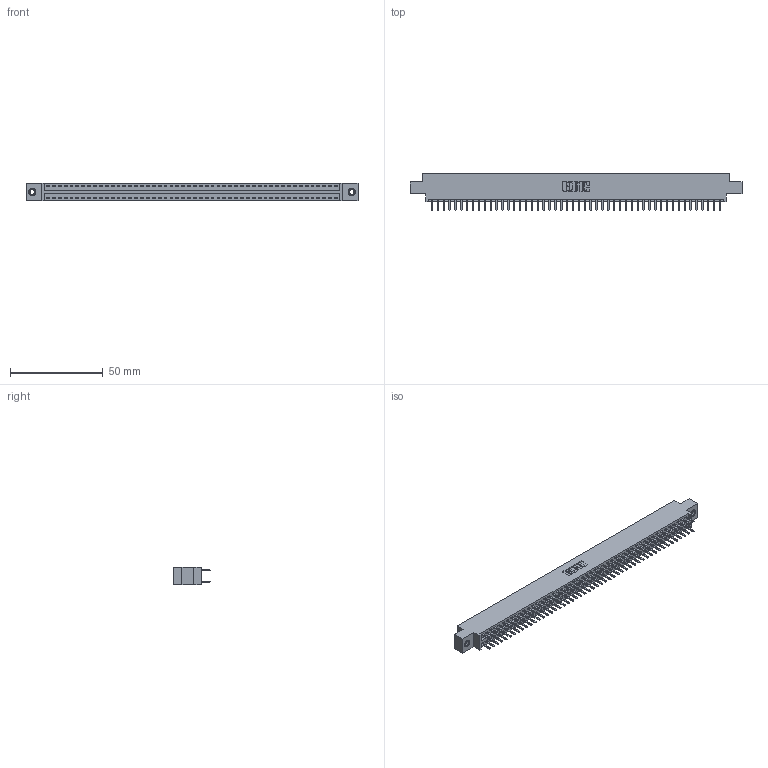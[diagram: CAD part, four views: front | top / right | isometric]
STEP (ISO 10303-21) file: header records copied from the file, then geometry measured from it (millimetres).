
FILE_DESCRIPTION (( 'STEP AP203' ), '1' );
FILE_NAME ('346-100-520-807.STEP', '2022-05-26T19:53:57', ( '' ), ( '' ), 'SwSTEP 2.0', 'SolidWorks 2020', '' );
FILE_SCHEMA (( 'CONFIG_CONTROL_DESIGN' ));
Length unit declared in the file: inch
Products named in the file (4): 345-292-001_345-293-120; 346-100-520-807; 345-250-001_345-250-005-103; 346 Part_0.170 Offset - 0.156 Dia-TI
Assembly tree (103 placements, depth 2):
  346-100-520-807
    346 Part_0.170 Offset - 0.156 Dia-TI
    345-292-001_345-293-120  x100
    345-250-001_345-250-005-103  x2
Bounding box: 179.32 x 20.02 x 9.4 mm (x, y, z)
Volume: 17336.4 mm3; surface area: 24066.1 mm2
Topology: 103 solids, 103 shells, 5786 faces, 16777 edges, 10910 vertices
Faces by surface type: plane 3812, cylinder 1958, cone 12, torus 4
Entity records: 32986 total; most frequent: CARTESIAN_POINT 5423, ORIENTED_EDGE 5338, DIRECTION 4843, EDGE_CURVE 2669, VECTOR 2313, LINE 2313, VERTEX_POINT 1772, AXIS2_PLACEMENT_3D 1265
